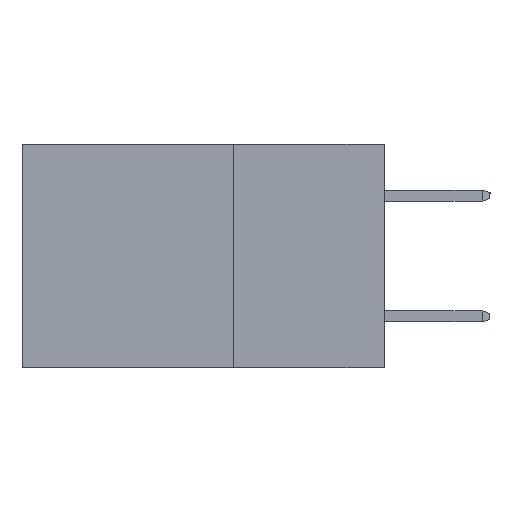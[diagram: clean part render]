
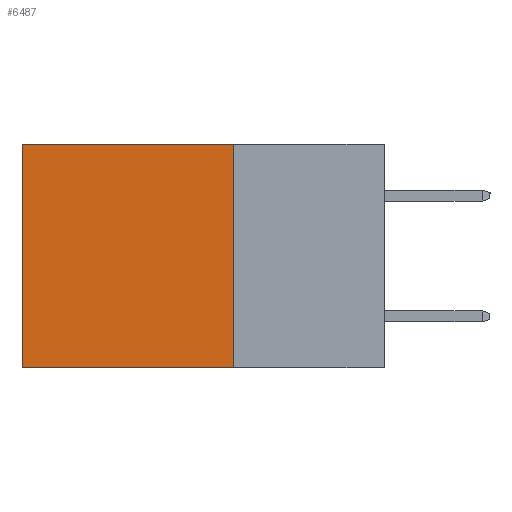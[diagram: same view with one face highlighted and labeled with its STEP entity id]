
A CAD part, left-side view. The second image highlights one B-rep face of the part: STEP entity #6487.
In plain terms, the highlighted planar face has unit normal (-1, 0, 0).
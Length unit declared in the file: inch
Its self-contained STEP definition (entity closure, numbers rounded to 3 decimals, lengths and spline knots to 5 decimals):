
#793 = PLANE ( 'NONE',  #7900 ) ;
#853 = DIRECTION ( 'NONE',  ( 0., 1., 0. ) ) ;
#1403 = VERTEX_POINT ( 'NONE', #7498 ) ;
#1452 = CARTESIAN_POINT ( 'NONE',  ( 0.2615, 0.25, -0.37 ) ) ;
#1805 = ORIENTED_EDGE ( 'NONE', *, *, #4580, .T. ) ;
#1931 = CARTESIAN_POINT ( 'NONE',  ( 0.2615, 0.6, 0. ) ) ;
#2368 = DIRECTION ( 'NONE',  ( 0., 0., -1. ) ) ;
#2509 = EDGE_CURVE ( 'NONE', #3420, #8505, #7181, .T. ) ;
#2521 = VECTOR ( 'NONE', #853, 39.37008 ) ;
#2992 = ORIENTED_EDGE ( 'NONE', *, *, #12282, .F. ) ;
#3190 = LINE ( 'NONE', #5248, #8892 ) ;
#3420 = VERTEX_POINT ( 'NONE', #1931 ) ;
#3547 = DIRECTION ( 'NONE',  ( 1., 0., 0. ) ) ;
#3704 = CARTESIAN_POINT ( 'NONE',  ( 0.2615, 0.6, -0.37 ) ) ;
#4130 = VECTOR ( 'NONE', #4273, 39.37008 ) ;
#4273 = DIRECTION ( 'NONE',  ( 0., 0., -1. ) ) ;
#4580 = EDGE_CURVE ( 'NONE', #1403, #3420, #3190, .T. ) ;
#4588 = CARTESIAN_POINT ( 'NONE',  ( 0.2615, 0.25, -0.37 ) ) ;
#4941 = ORIENTED_EDGE ( 'NONE', *, *, #2509, .T. ) ;
#5248 = CARTESIAN_POINT ( 'NONE',  ( 0.2615, 0.25, 0. ) ) ;
#6459 = FACE_OUTER_BOUND ( 'NONE', #11643, .T. ) ;
#6487 = ADVANCED_FACE ( 'NONE', ( #6459 ), #793, .F. ) ;
#6659 = LINE ( 'NONE', #4588, #2521 ) ;
#7181 = LINE ( 'NONE', #8158, #4130 ) ;
#7498 = CARTESIAN_POINT ( 'NONE',  ( 0.2615, 0.25, 0. ) ) ;
#7900 = AXIS2_PLACEMENT_3D ( 'NONE', #11598, #3547, #10388 ) ;
#8158 = CARTESIAN_POINT ( 'NONE',  ( 0.2615, 0.6, -0.37 ) ) ;
#8505 = VERTEX_POINT ( 'NONE', #3704 ) ;
#8892 = VECTOR ( 'NONE', #9185, 39.37008 ) ;
#9185 = DIRECTION ( 'NONE',  ( 0., 1., 0. ) ) ;
#9509 = VECTOR ( 'NONE', #2368, 39.37008 ) ;
#10208 = CARTESIAN_POINT ( 'NONE',  ( 0.2615, 0.25, -0.37 ) ) ;
#10388 = DIRECTION ( 'NONE',  ( 0., 0., -1. ) ) ;
#10402 = EDGE_CURVE ( 'NONE', #1403, #10842, #11252, .T. ) ;
#10842 = VERTEX_POINT ( 'NONE', #10208 ) ;
#11252 = LINE ( 'NONE', #1452, #9509 ) ;
#11598 = CARTESIAN_POINT ( 'NONE',  ( 0.2615, 0.25, -0.37 ) ) ;
#11643 = EDGE_LOOP ( 'NONE', ( #4941, #2992, #12423, #1805 ) ) ;
#12282 = EDGE_CURVE ( 'NONE', #10842, #8505, #6659, .T. ) ;
#12423 = ORIENTED_EDGE ( 'NONE', *, *, #10402, .F. ) ;
